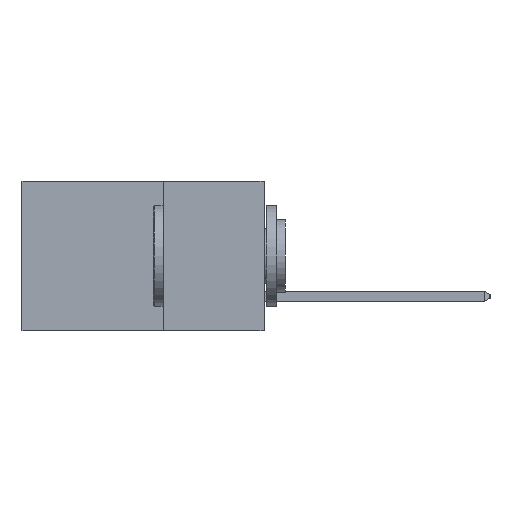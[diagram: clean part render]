
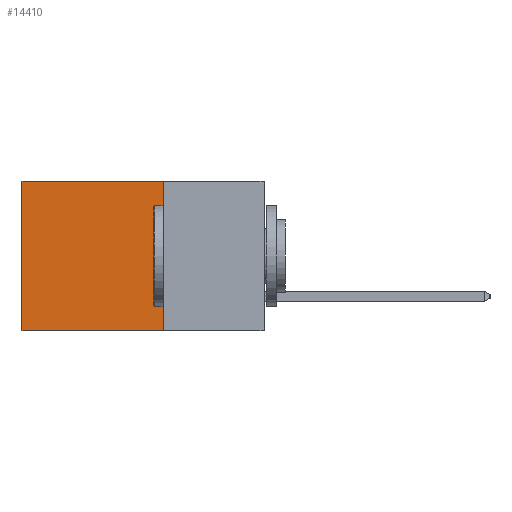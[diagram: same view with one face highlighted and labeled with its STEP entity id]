
A CAD part, left-side view. The second image highlights one B-rep face of the part: STEP entity #14410.
In plain terms, the highlighted planar face has unit normal (-1, 0, 0).
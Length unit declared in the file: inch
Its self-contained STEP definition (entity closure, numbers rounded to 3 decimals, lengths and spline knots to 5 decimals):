
#858 = VECTOR ( 'NONE', #10429, 39.37008 ) ;
#947 = CARTESIAN_POINT ( 'NONE',  ( 0.298, 0.6, -0.37 ) ) ;
#974 = CARTESIAN_POINT ( 'NONE',  ( 0.298, 0.25, 0. ) ) ;
#2433 = CARTESIAN_POINT ( 'NONE',  ( 0.298, 0.25, -0.37 ) ) ;
#3049 = PLANE ( 'NONE',  #9643 ) ;
#3182 = VERTEX_POINT ( 'NONE', #974 ) ;
#3434 = EDGE_CURVE ( 'NONE', #3182, #3516, #4876, .T. ) ;
#3516 = VERTEX_POINT ( 'NONE', #3967 ) ;
#3967 = CARTESIAN_POINT ( 'NONE',  ( 0.298, 0.25, -0.37 ) ) ;
#4114 = CARTESIAN_POINT ( 'NONE',  ( 0.298, 0.25, 0. ) ) ;
#4167 = ORIENTED_EDGE ( 'NONE', *, *, #14017, .F. ) ;
#4195 = DIRECTION ( 'NONE',  ( 1., 0., 0. ) ) ;
#4675 = EDGE_CURVE ( 'NONE', #6899, #12172, #14948, .T. ) ;
#4767 = ORIENTED_EDGE ( 'NONE', *, *, #7876, .T. ) ;
#4876 = LINE ( 'NONE', #4114, #8159 ) ;
#5256 = ORIENTED_EDGE ( 'NONE', *, *, #3434, .F. ) ;
#5591 = DIRECTION ( 'NONE',  ( 0., 0., -1. ) ) ;
#6617 = CARTESIAN_POINT ( 'NONE',  ( 0.298, 0.25, 0. ) ) ;
#6899 = VERTEX_POINT ( 'NONE', #7639 ) ;
#7639 = CARTESIAN_POINT ( 'NONE',  ( 0.298, 0.6, 0. ) ) ;
#7794 = ORIENTED_EDGE ( 'NONE', *, *, #4675, .T. ) ;
#7876 = EDGE_CURVE ( 'NONE', #3182, #6899, #10370, .T. ) ;
#8159 = VECTOR ( 'NONE', #11443, 39.37008 ) ;
#9179 = VECTOR ( 'NONE', #5591, 39.37008 ) ;
#9612 = DIRECTION ( 'NONE',  ( 0., 1., 0. ) ) ;
#9643 = AXIS2_PLACEMENT_3D ( 'NONE', #6617, #4195, #12429 ) ;
#9766 = FACE_OUTER_BOUND ( 'NONE', #11469, .T. ) ;
#10370 = LINE ( 'NONE', #12685, #858 ) ;
#10429 = DIRECTION ( 'NONE',  ( 0., 1., 0. ) ) ;
#11443 = DIRECTION ( 'NONE',  ( 0., 0., -1. ) ) ;
#11469 = EDGE_LOOP ( 'NONE', ( #7794, #4167, #5256, #4767 ) ) ;
#11715 = LINE ( 'NONE', #2433, #14445 ) ;
#12172 = VERTEX_POINT ( 'NONE', #947 ) ;
#12429 = DIRECTION ( 'NONE',  ( 0., 0., -1. ) ) ;
#12685 = CARTESIAN_POINT ( 'NONE',  ( 0.298, 0.25, 0. ) ) ;
#12765 = CARTESIAN_POINT ( 'NONE',  ( 0.298, 0.6, 0. ) ) ;
#14017 = EDGE_CURVE ( 'NONE', #3516, #12172, #11715, .T. ) ;
#14410 = ADVANCED_FACE ( 'NONE', ( #9766 ), #3049, .F. ) ;
#14445 = VECTOR ( 'NONE', #9612, 39.37008 ) ;
#14948 = LINE ( 'NONE', #12765, #9179 ) ;
